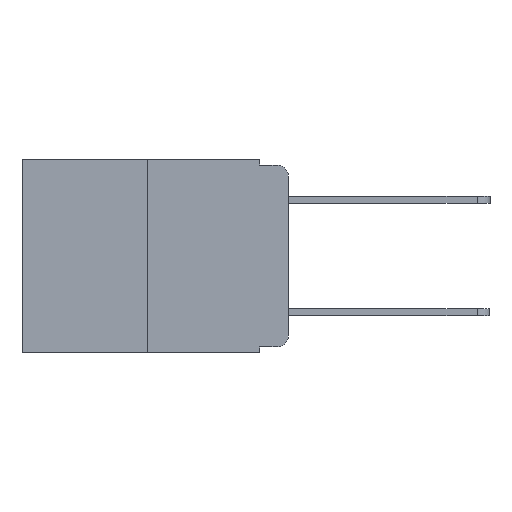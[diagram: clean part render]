
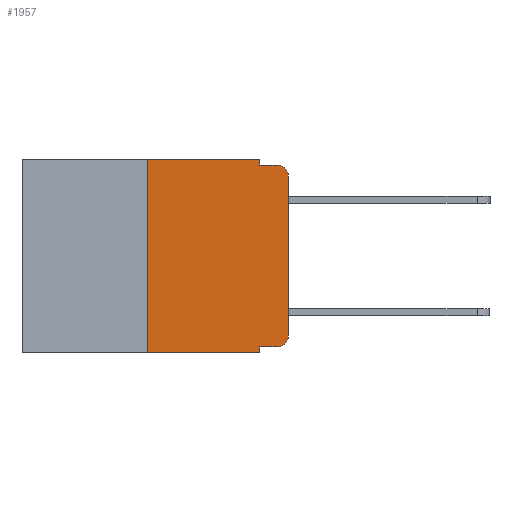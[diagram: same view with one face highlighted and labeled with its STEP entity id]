
A CAD part, left-side view. The second image highlights one B-rep face of the part: STEP entity #1957.
In plain terms, the highlighted planar face has unit normal (-1, 0, 0).
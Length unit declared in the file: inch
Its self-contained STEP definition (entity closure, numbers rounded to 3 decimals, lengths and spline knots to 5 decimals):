
#172 = AXIS2_PLACEMENT_3D ( 'NONE', #2074, #4842, #4792 ) ;
#283 = CARTESIAN_POINT ( 'NONE',  ( 0., 0.051, -0.333 ) ) ;
#317 = VERTEX_POINT ( 'NONE', #10743 ) ;
#468 = DIRECTION ( 'NONE',  ( 0., 0., 1. ) ) ;
#623 = VERTEX_POINT ( 'NONE', #8201 ) ;
#1169 = VERTEX_POINT ( 'NONE', #11920 ) ;
#1305 = EDGE_CURVE ( 'NONE', #10562, #5096, #8992, .T. ) ;
#1687 = CARTESIAN_POINT ( 'NONE',  ( 0., 0.473, 0. ) ) ;
#1858 = ORIENTED_EDGE ( 'NONE', *, *, #2848, .T. ) ;
#1874 = ORIENTED_EDGE ( 'NONE', *, *, #2896, .F. ) ;
#1957 = ADVANCED_FACE ( 'NONE', ( #11785 ), #6011, .F. ) ;
#2074 = CARTESIAN_POINT ( 'NONE',  ( 0., 0.02, -0.313 ) ) ;
#2147 = EDGE_CURVE ( 'NONE', #10576, #317, #11125, .T. ) ;
#2217 = VERTEX_POINT ( 'NONE', #3322 ) ;
#2631 = ORIENTED_EDGE ( 'NONE', *, *, #2871, .T. ) ;
#2848 = EDGE_CURVE ( 'NONE', #1169, #2217, #4037, .T. ) ;
#2871 = EDGE_CURVE ( 'NONE', #2217, #6182, #11083, .T. ) ;
#2876 = EDGE_CURVE ( 'NONE', #623, #6182, #3299, .T. ) ;
#2893 = EDGE_CURVE ( 'NONE', #5096, #623, #5627, .T. ) ;
#2894 = EDGE_CURVE ( 'NONE', #10576, #10562, #12572, .T. ) ;
#2896 = EDGE_CURVE ( 'NONE', #13164, #317, #12847, .T. ) ;
#2910 = EDGE_CURVE ( 'NONE', #13164, #10951, #9971, .T. ) ;
#2915 = VECTOR ( 'NONE', #6734, 39.37008 ) ;
#3056 = EDGE_CURVE ( 'NONE', #10951, #1169, #7162, .T. ) ;
#3299 = LINE ( 'NONE', #8212, #2915 ) ;
#3322 = CARTESIAN_POINT ( 'NONE',  ( 0., 0., -0.03 ) ) ;
#4037 = LINE ( 'NONE', #6643, #7173 ) ;
#4421 = CARTESIAN_POINT ( 'NONE',  ( 0., 0.02, -0.333 ) ) ;
#4431 = CARTESIAN_POINT ( 'NONE',  ( 0., 0.051, -0.333 ) ) ;
#4555 = AXIS2_PLACEMENT_3D ( 'NONE', #5789, #5737, #5703 ) ;
#4661 = CARTESIAN_POINT ( 'NONE',  ( 0., 0.25, 0. ) ) ;
#4792 = DIRECTION ( 'NONE',  ( 0., 0., -1. ) ) ;
#4842 = DIRECTION ( 'NONE',  ( -1., 0., 0. ) ) ;
#5096 = VERTEX_POINT ( 'NONE', #7886 ) ;
#5627 = LINE ( 'NONE', #9264, #7890 ) ;
#5703 = DIRECTION ( 'NONE',  ( 0., 0., -1. ) ) ;
#5711 = ORIENTED_EDGE ( 'NONE', *, *, #1305, .F. ) ;
#5737 = DIRECTION ( 'NONE',  ( 1., 0., 0. ) ) ;
#5789 = CARTESIAN_POINT ( 'NONE',  ( 0., 0.473, 0. ) ) ;
#5858 = DIRECTION ( 'NONE',  ( 0., -1., 0. ) ) ;
#5891 = CARTESIAN_POINT ( 'NONE',  ( 0., 0.25, 0. ) ) ;
#5911 = VECTOR ( 'NONE', #5858, 39.37008 ) ;
#6011 = PLANE ( 'NONE',  #4555 ) ;
#6182 = VERTEX_POINT ( 'NONE', #10110 ) ;
#6643 = CARTESIAN_POINT ( 'NONE',  ( 0., 0., 0. ) ) ;
#6734 = DIRECTION ( 'NONE',  ( 0., -1., 0. ) ) ;
#6903 = CARTESIAN_POINT ( 'NONE',  ( 0., 0.25, -0.343 ) ) ;
#6929 = DIRECTION ( 'NONE',  ( 0., 0., -1. ) ) ;
#6945 = EDGE_LOOP ( 'NONE', ( #1858, #2631, #7964, #10584, #5711, #8536, #12915, #1874, #10859, #8808 ) ) ;
#7162 = CIRCLE ( 'NONE', #172, 0.02 ) ;
#7173 = VECTOR ( 'NONE', #12522, 39.37008 ) ;
#7391 = DIRECTION ( 'NONE',  ( 0., -1., 0. ) ) ;
#7886 = CARTESIAN_POINT ( 'NONE',  ( 0., 0.051, 0. ) ) ;
#7890 = VECTOR ( 'NONE', #9864, 39.37008 ) ;
#7964 = ORIENTED_EDGE ( 'NONE', *, *, #2876, .F. ) ;
#8113 = DIRECTION ( 'NONE',  ( -1., 0., 0. ) ) ;
#8201 = CARTESIAN_POINT ( 'NONE',  ( 0., 0.051, -0.01 ) ) ;
#8212 = CARTESIAN_POINT ( 'NONE',  ( 0., 0.051, -0.01 ) ) ;
#8536 = ORIENTED_EDGE ( 'NONE', *, *, #2894, .F. ) ;
#8808 = ORIENTED_EDGE ( 'NONE', *, *, #3056, .T. ) ;
#8992 = LINE ( 'NONE', #1687, #5911 ) ;
#9264 = CARTESIAN_POINT ( 'NONE',  ( 0., 0.051, 0. ) ) ;
#9698 = VECTOR ( 'NONE', #7391, 39.37008 ) ;
#9864 = DIRECTION ( 'NONE',  ( 0., 0., -1. ) ) ;
#9916 = CARTESIAN_POINT ( 'NONE',  ( 0., 0.051, 0. ) ) ;
#9971 = LINE ( 'NONE', #4431, #9698 ) ;
#10110 = CARTESIAN_POINT ( 'NONE',  ( 0., 0.02, -0.01 ) ) ;
#10236 = VECTOR ( 'NONE', #468, 39.37008 ) ;
#10240 = CARTESIAN_POINT ( 'NONE',  ( 0., 0.473, -0.343 ) ) ;
#10562 = VERTEX_POINT ( 'NONE', #5891 ) ;
#10576 = VERTEX_POINT ( 'NONE', #6903 ) ;
#10584 = ORIENTED_EDGE ( 'NONE', *, *, #2893, .F. ) ;
#10627 = DIRECTION ( 'NONE',  ( 0., -1., 0. ) ) ;
#10743 = CARTESIAN_POINT ( 'NONE',  ( 0., 0.051, -0.343 ) ) ;
#10758 = DIRECTION ( 'NONE',  ( 0., 0., -1. ) ) ;
#10827 = VECTOR ( 'NONE', #10627, 39.37008 ) ;
#10859 = ORIENTED_EDGE ( 'NONE', *, *, #2910, .T. ) ;
#10951 = VERTEX_POINT ( 'NONE', #4421 ) ;
#11083 = CIRCLE ( 'NONE', #12927, 0.02 ) ;
#11125 = LINE ( 'NONE', #10240, #10827 ) ;
#11785 = FACE_OUTER_BOUND ( 'NONE', #6945, .T. ) ;
#11920 = CARTESIAN_POINT ( 'NONE',  ( 0., 0., -0.313 ) ) ;
#12302 = VECTOR ( 'NONE', #10758, 39.37008 ) ;
#12522 = DIRECTION ( 'NONE',  ( 0., 0., 1. ) ) ;
#12572 = LINE ( 'NONE', #4661, #10236 ) ;
#12655 = CARTESIAN_POINT ( 'NONE',  ( 0., 0.02, -0.03 ) ) ;
#12847 = LINE ( 'NONE', #9916, #12302 ) ;
#12915 = ORIENTED_EDGE ( 'NONE', *, *, #2147, .T. ) ;
#12927 = AXIS2_PLACEMENT_3D ( 'NONE', #12655, #8113, #6929 ) ;
#13164 = VERTEX_POINT ( 'NONE', #283 ) ;
